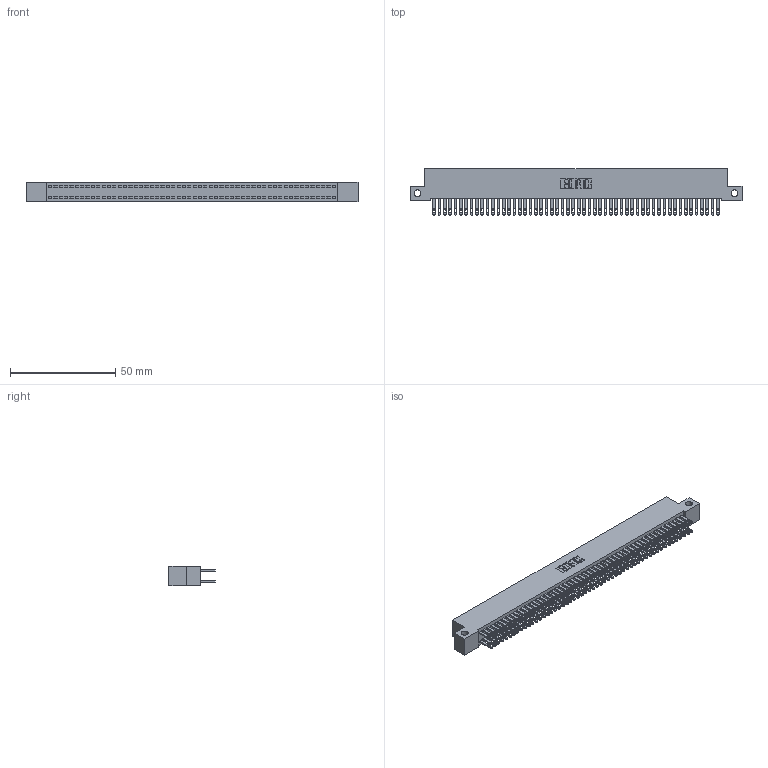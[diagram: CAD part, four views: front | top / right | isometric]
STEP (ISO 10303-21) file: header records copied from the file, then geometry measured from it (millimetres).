
FILE_DESCRIPTION (( 'STEP AP203' ), '1' );
FILE_NAME ('342-108-500-212.STEP', '2018-08-14T07:29:55', ( '' ), ( '' ), 'SwSTEP 2.0', 'SolidWorks 2016', '' );
FILE_SCHEMA (( 'CONFIG_CONTROL_DESIGN' ));
Length unit declared in the file: inch
Products named in the file (3): 345-292-001_345-293-100; 342-108-500-212; 342 Part_Side Mount
Assembly tree (109 placements, depth 2):
  342-108-500-212
    342 Part_Side Mount
    345-292-001_345-293-100  x108
Bounding box: 157.48 x 21.85 x 9.4 mm (x, y, z)
Volume: 14462.5 mm3; surface area: 24711.2 mm2
Topology: 109 solids, 109 shells, 5294 faces, 16175 edges, 10782 vertices
Faces by surface type: plane 3306, cylinder 1988
Entity records: 32989 total; most frequent: CARTESIAN_POINT 5450, ORIENTED_EDGE 5386, DIRECTION 4637, EDGE_CURVE 2693, VECTOR 2561, LINE 2561, VERTEX_POINT 1794, AXIS2_PLACEMENT_3D 1038
